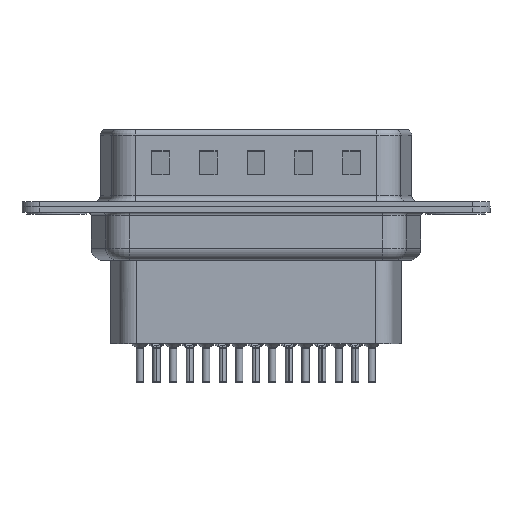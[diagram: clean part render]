
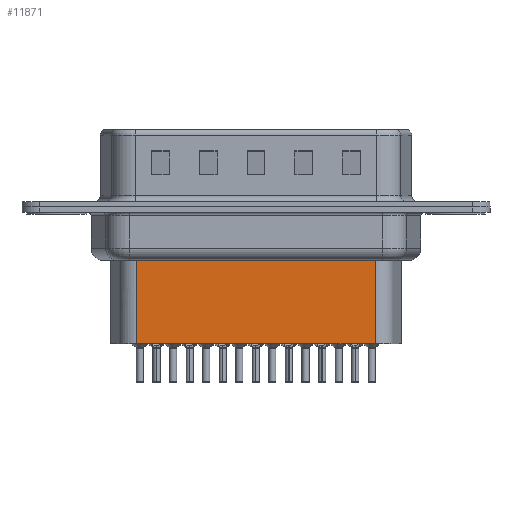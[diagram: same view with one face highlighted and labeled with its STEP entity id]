
A CAD part, front view. The second image highlights one B-rep face of the part: STEP entity #11871.
In plain terms, the highlighted planar face has unit normal (0, -1, 0).
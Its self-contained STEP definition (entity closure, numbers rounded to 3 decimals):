
#421 = AXIS2_PLACEMENT_3D ( 'NONE', #6807, #17392, #8327 ) ;
#1164 = VECTOR ( 'NONE', #8370, 1000. ) ;
#1543 = CARTESIAN_POINT ( 'NONE',  ( 6.681, -3.5, -4.097 ) ) ;
#1895 = EDGE_CURVE ( 'NONE', #2965, #18662, #4327, .T. ) ;
#2077 = CARTESIAN_POINT ( 'NONE',  ( 26.619, -3.5, -3.1 ) ) ;
#2112 = LINE ( 'NONE', #2077, #17672 ) ;
#2609 = ORIENTED_EDGE ( 'NONE', *, *, #16404, .F. ) ;
#2965 = VERTEX_POINT ( 'NONE', #4196 ) ;
#3467 = LINE ( 'NONE', #18212, #11467 ) ;
#4196 = CARTESIAN_POINT ( 'NONE',  ( 26.619, -3.5, -11.45 ) ) ;
#4327 = LINE ( 'NONE', #11290, #15900 ) ;
#6004 = CARTESIAN_POINT ( 'NONE',  ( 6.681, -3.5, -11.45 ) ) ;
#6131 = VERTEX_POINT ( 'NONE', #11251 ) ;
#6807 = CARTESIAN_POINT ( 'NONE',  ( 6.681, -3.5, -3.1 ) ) ;
#8096 = DIRECTION ( 'NONE',  ( 0., 0., -1. ) ) ;
#8327 = DIRECTION ( 'NONE',  ( 1., 0., 0. ) ) ;
#8370 = DIRECTION ( 'NONE',  ( -1., 0., 0. ) ) ;
#8528 = ORIENTED_EDGE ( 'NONE', *, *, #15901, .T. ) ;
#10537 = VERTEX_POINT ( 'NONE', #1543 ) ;
#10577 = EDGE_CURVE ( 'NONE', #10537, #18662, #3467, .T. ) ;
#11070 = DIRECTION ( 'NONE',  ( -1., 0., 0. ) ) ;
#11251 = CARTESIAN_POINT ( 'NONE',  ( 26.619, -3.5, -4.097 ) ) ;
#11290 = CARTESIAN_POINT ( 'NONE',  ( 6.681, -3.5, -11.45 ) ) ;
#11453 = FACE_OUTER_BOUND ( 'NONE', #13686, .T. ) ;
#11467 = VECTOR ( 'NONE', #16704, 1000. ) ;
#11871 = ADVANCED_FACE ( 'NONE', ( #11453 ), #12730, .T. ) ;
#12730 = PLANE ( 'NONE',  #421 ) ;
#13686 = EDGE_LOOP ( 'NONE', ( #2609, #8528, #14681, #16449 ) ) ;
#14388 = CARTESIAN_POINT ( 'NONE',  ( 6.434, -3.5, -4.097 ) ) ;
#14681 = ORIENTED_EDGE ( 'NONE', *, *, #10577, .T. ) ;
#15900 = VECTOR ( 'NONE', #11070, 1000. ) ;
#15901 = EDGE_CURVE ( 'NONE', #6131, #10537, #17217, .T. ) ;
#16404 = EDGE_CURVE ( 'NONE', #6131, #2965, #2112, .T. ) ;
#16449 = ORIENTED_EDGE ( 'NONE', *, *, #1895, .F. ) ;
#16704 = DIRECTION ( 'NONE',  ( 0., 0., -1. ) ) ;
#17217 = LINE ( 'NONE', #14388, #1164 ) ;
#17392 = DIRECTION ( 'NONE',  ( 0., -1., 0. ) ) ;
#17672 = VECTOR ( 'NONE', #8096, 1000. ) ;
#18212 = CARTESIAN_POINT ( 'NONE',  ( 6.681, -3.5, -3.1 ) ) ;
#18662 = VERTEX_POINT ( 'NONE', #6004 ) ;
